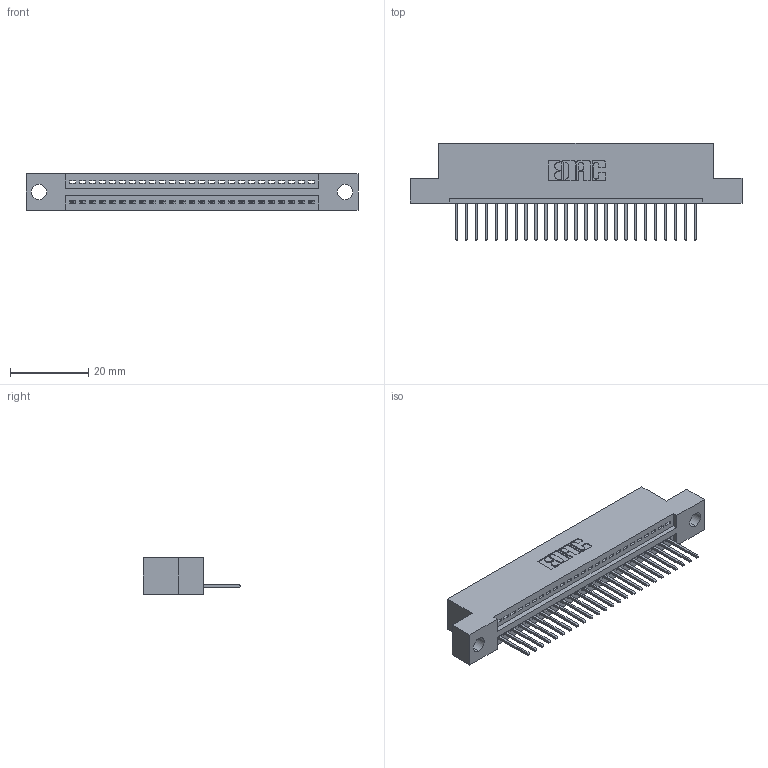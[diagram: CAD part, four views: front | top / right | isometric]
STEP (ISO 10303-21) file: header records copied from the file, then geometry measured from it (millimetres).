
FILE_DESCRIPTION (( 'STEP AP203' ), '1' );
FILE_NAME ('345-025-523-104.STEP', '2021-05-26T14:29:27', ( '' ), ( '' ), 'SwSTEP 2.0', 'SolidWorks 2020', '' );
FILE_SCHEMA (( 'CONFIG_CONTROL_DESIGN' ));
Length unit declared in the file: inch
Products named in the file (3): 345-292-001_345-293-123; 345 Part_Flush Mounting Lugs - 0.156 Dia-TI; 345-025-523-104
Assembly tree (26 placements, depth 2):
  345-025-523-104
    345 Part_Flush Mounting Lugs - 0.156 Dia-TI
    345-292-001_345-293-123  x25
Bounding box: 84.71 x 24.82 x 9.4 mm (x, y, z)
Volume: 7790.9 mm3; surface area: 9992 mm2
Topology: 26 solids, 26 shells, 1590 faces, 4777 edges, 3150 vertices
Faces by surface type: plane 1094, cylinder 496
Entity records: 21541 total; most frequent: CARTESIAN_POINT 3741, ORIENTED_EDGE 3698, DIRECTION 3291, EDGE_CURVE 1849, VECTOR 1617, LINE 1617, VERTEX_POINT 1230, AXIS2_PLACEMENT_3D 837
